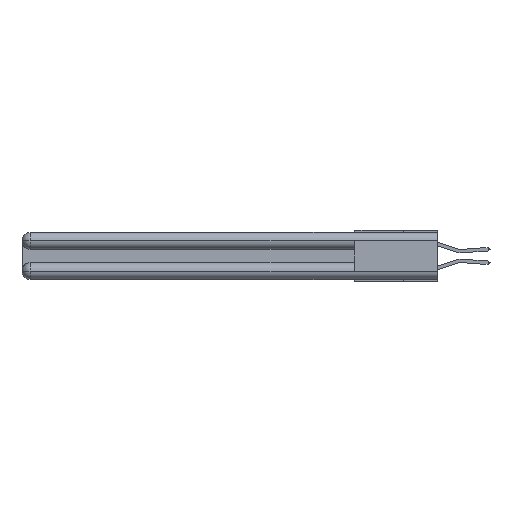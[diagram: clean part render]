
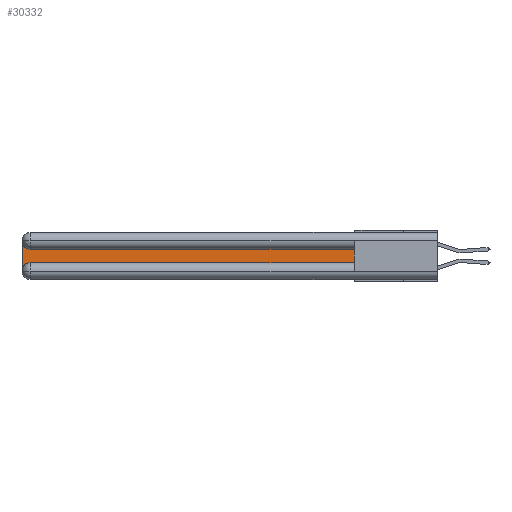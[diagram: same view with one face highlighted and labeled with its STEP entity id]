
A CAD part, left-side view. The second image highlights one B-rep face of the part: STEP entity #30332.
In plain terms, the highlighted planar face has unit normal (-1, 0, 0).
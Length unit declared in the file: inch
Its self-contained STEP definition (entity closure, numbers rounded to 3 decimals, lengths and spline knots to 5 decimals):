
#32 = CARTESIAN_POINT ( 'NONE',  ( 0.075, 2.94, -0.2175 ) ) ;
#966 = CARTESIAN_POINT ( 'NONE',  ( 0.075, 0.6, -0.2175 ) ) ;
#2968 = CARTESIAN_POINT ( 'NONE',  ( 0.075, 3., -0.2175 ) ) ;
#3075 = CARTESIAN_POINT ( 'NONE',  ( 0.075, 2.94, -0.0625 ) ) ;
#3416 = EDGE_CURVE ( 'NONE', #29784, #20018, #5466, .T. ) ;
#4609 = CARTESIAN_POINT ( 'NONE',  ( 0.075, 3., -0.1225 ) ) ;
#5466 = LINE ( 'NONE', #17213, #6329 ) ;
#5732 = VERTEX_POINT ( 'NONE', #6789 ) ;
#6329 = VECTOR ( 'NONE', #16879, 39.37008 ) ;
#6789 = CARTESIAN_POINT ( 'NONE',  ( 0.075, 3., -0.0625 ) ) ;
#6790 = CIRCLE ( 'NONE', #15891, 0.06 ) ;
#7880 = DIRECTION ( 'NONE',  ( 0., 0., -1. ) ) ;
#8090 = DIRECTION ( 'NONE',  ( 0., 0., -1. ) ) ;
#8165 = LINE ( 'NONE', #2968, #14219 ) ;
#8414 = VECTOR ( 'NONE', #14117, 39.37008 ) ;
#8486 = AXIS2_PLACEMENT_3D ( 'NONE', #28817, #20796, #8090 ) ;
#8540 = DIRECTION ( 'NONE',  ( 0., 1., 0. ) ) ;
#9510 = ORIENTED_EDGE ( 'NONE', *, *, #3416, .T. ) ;
#10771 = CARTESIAN_POINT ( 'NONE',  ( 0.075, 0.6, -0.1225 ) ) ;
#11765 = ORIENTED_EDGE ( 'NONE', *, *, #17089, .T. ) ;
#12288 = FACE_OUTER_BOUND ( 'NONE', #23620, .T. ) ;
#12985 = EDGE_CURVE ( 'NONE', #33337, #22219, #22230, .T. ) ;
#13117 = VERTEX_POINT ( 'NONE', #16025 ) ;
#14117 = DIRECTION ( 'NONE',  ( 0., 0., 1. ) ) ;
#14205 = CIRCLE ( 'NONE', #8486, 0.06 ) ;
#14219 = VECTOR ( 'NONE', #31384, 39.37008 ) ;
#15891 = AXIS2_PLACEMENT_3D ( 'NONE', #3075, #28849, #18120 ) ;
#16025 = CARTESIAN_POINT ( 'NONE',  ( 0.075, 3., -0.2775 ) ) ;
#16879 = DIRECTION ( 'NONE',  ( 0., -1., 0. ) ) ;
#17089 = EDGE_CURVE ( 'NONE', #20018, #33337, #25400, .T. ) ;
#17213 = CARTESIAN_POINT ( 'NONE',  ( 0.075, 0.6, -0.2175 ) ) ;
#17369 = CARTESIAN_POINT ( 'NONE',  ( 0.075, 2.94, -0.1225 ) ) ;
#18120 = DIRECTION ( 'NONE',  ( 0., 0., -1. ) ) ;
#19836 = ORIENTED_EDGE ( 'NONE', *, *, #24509, .T. ) ;
#20018 = VERTEX_POINT ( 'NONE', #30369 ) ;
#20796 = DIRECTION ( 'NONE',  ( 1., 0., 0. ) ) ;
#21178 = ORIENTED_EDGE ( 'NONE', *, *, #32701, .T. ) ;
#21812 = VECTOR ( 'NONE', #8540, 39.37008 ) ;
#22219 = VERTEX_POINT ( 'NONE', #17369 ) ;
#22230 = LINE ( 'NONE', #24135, #21812 ) ;
#22377 = EDGE_CURVE ( 'NONE', #5732, #13117, #8165, .T. ) ;
#22495 = PLANE ( 'NONE',  #23367 ) ;
#22722 = DIRECTION ( 'NONE',  ( 1., 0., 0. ) ) ;
#23367 = AXIS2_PLACEMENT_3D ( 'NONE', #4609, #22722, #7880 ) ;
#23620 = EDGE_LOOP ( 'NONE', ( #27524, #19836, #26700, #21178, #9510, #11765 ) ) ;
#24135 = CARTESIAN_POINT ( 'NONE',  ( 0.075, 0.6, -0.1225 ) ) ;
#24509 = EDGE_CURVE ( 'NONE', #22219, #5732, #6790, .T. ) ;
#25400 = LINE ( 'NONE', #966, #8414 ) ;
#26700 = ORIENTED_EDGE ( 'NONE', *, *, #22377, .T. ) ;
#27524 = ORIENTED_EDGE ( 'NONE', *, *, #12985, .T. ) ;
#28817 = CARTESIAN_POINT ( 'NONE',  ( 0.075, 2.94, -0.2775 ) ) ;
#28849 = DIRECTION ( 'NONE',  ( 1., 0., 0. ) ) ;
#29784 = VERTEX_POINT ( 'NONE', #32 ) ;
#30332 = ADVANCED_FACE ( 'NONE', ( #12288 ), #22495, .F. ) ;
#30369 = CARTESIAN_POINT ( 'NONE',  ( 0.075, 0.6, -0.2175 ) ) ;
#31384 = DIRECTION ( 'NONE',  ( 0., 0., -1. ) ) ;
#32701 = EDGE_CURVE ( 'NONE', #13117, #29784, #14205, .T. ) ;
#33337 = VERTEX_POINT ( 'NONE', #10771 ) ;
